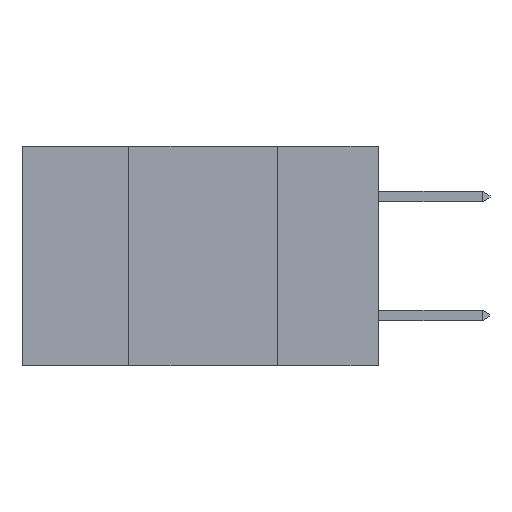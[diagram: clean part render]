
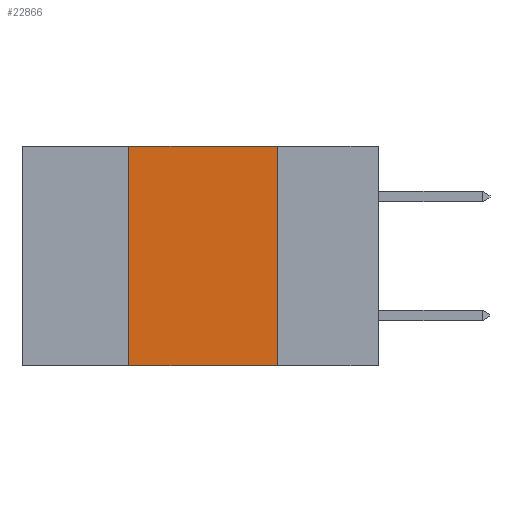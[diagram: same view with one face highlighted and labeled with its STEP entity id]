
A CAD part, left-side view. The second image highlights one B-rep face of the part: STEP entity #22866.
In plain terms, the highlighted planar face has unit normal (-1, 0, 0).
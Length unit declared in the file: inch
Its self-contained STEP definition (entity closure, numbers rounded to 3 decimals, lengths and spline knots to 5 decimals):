
#1300 = VECTOR ( 'NONE', #2633, 39.37008 ) ;
#1664 = ORIENTED_EDGE ( 'NONE', *, *, #16576, .F. ) ;
#2633 = DIRECTION ( 'NONE',  ( 0., -1., 0. ) ) ;
#3028 = CARTESIAN_POINT ( 'NONE',  ( 0., 0.42, 0. ) ) ;
#3375 = VERTEX_POINT ( 'NONE', #19997 ) ;
#4422 = CARTESIAN_POINT ( 'NONE',  ( 0., 0.42, -0.37 ) ) ;
#4756 = LINE ( 'NONE', #12516, #9797 ) ;
#5616 = DIRECTION ( 'NONE',  ( 0., 0., -1. ) ) ;
#6164 = VECTOR ( 'NONE', #8294, 39.37008 ) ;
#6694 = ORIENTED_EDGE ( 'NONE', *, *, #9933, .F. ) ;
#7666 = VERTEX_POINT ( 'NONE', #4422 ) ;
#7823 = ORIENTED_EDGE ( 'NONE', *, *, #11177, .F. ) ;
#7905 = AXIS2_PLACEMENT_3D ( 'NONE', #15037, #16907, #5616 ) ;
#8294 = DIRECTION ( 'NONE',  ( 0., 0., 1. ) ) ;
#9797 = VECTOR ( 'NONE', #16314, 39.37008 ) ;
#9933 = EDGE_CURVE ( 'NONE', #7666, #18003, #15035, .T. ) ;
#11177 = EDGE_CURVE ( 'NONE', #19203, #3375, #17904, .T. ) ;
#11326 = LINE ( 'NONE', #15835, #1300 ) ;
#12516 = CARTESIAN_POINT ( 'NONE',  ( 0., 0.6, -0.37 ) ) ;
#12837 = ORIENTED_EDGE ( 'NONE', *, *, #14706, .T. ) ;
#13124 = PLANE ( 'NONE',  #7905 ) ;
#14324 = FACE_OUTER_BOUND ( 'NONE', #23292, .T. ) ;
#14706 = EDGE_CURVE ( 'NONE', #7666, #3375, #4756, .T. ) ;
#15035 = LINE ( 'NONE', #19527, #6164 ) ;
#15037 = CARTESIAN_POINT ( 'NONE',  ( 0., 0.6, 0. ) ) ;
#15835 = CARTESIAN_POINT ( 'NONE',  ( 0., 0.6, 0. ) ) ;
#16314 = DIRECTION ( 'NONE',  ( 0., -1., 0. ) ) ;
#16576 = EDGE_CURVE ( 'NONE', #18003, #19203, #11326, .T. ) ;
#16907 = DIRECTION ( 'NONE',  ( 1., 0., 0. ) ) ;
#17904 = LINE ( 'NONE', #18822, #18456 ) ;
#18003 = VERTEX_POINT ( 'NONE', #3028 ) ;
#18456 = VECTOR ( 'NONE', #18894, 39.37008 ) ;
#18822 = CARTESIAN_POINT ( 'NONE',  ( 0., 0.17, 0. ) ) ;
#18894 = DIRECTION ( 'NONE',  ( 0., 0., -1. ) ) ;
#19203 = VERTEX_POINT ( 'NONE', #20570 ) ;
#19527 = CARTESIAN_POINT ( 'NONE',  ( 0., 0.42, 0. ) ) ;
#19997 = CARTESIAN_POINT ( 'NONE',  ( 0., 0.17, -0.37 ) ) ;
#20570 = CARTESIAN_POINT ( 'NONE',  ( 0., 0.17, 0. ) ) ;
#22866 = ADVANCED_FACE ( 'NONE', ( #14324 ), #13124, .F. ) ;
#23292 = EDGE_LOOP ( 'NONE', ( #7823, #1664, #6694, #12837 ) ) ;
